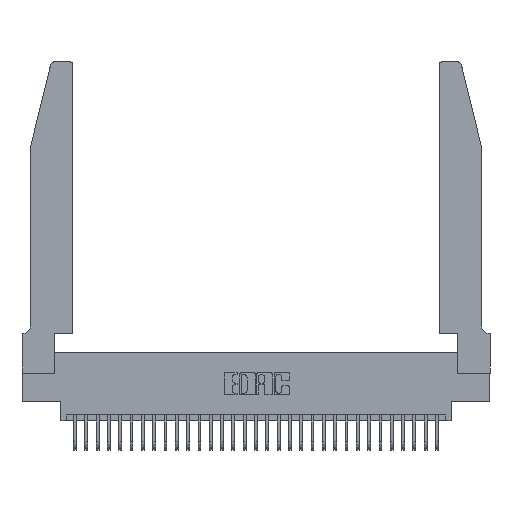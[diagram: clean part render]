
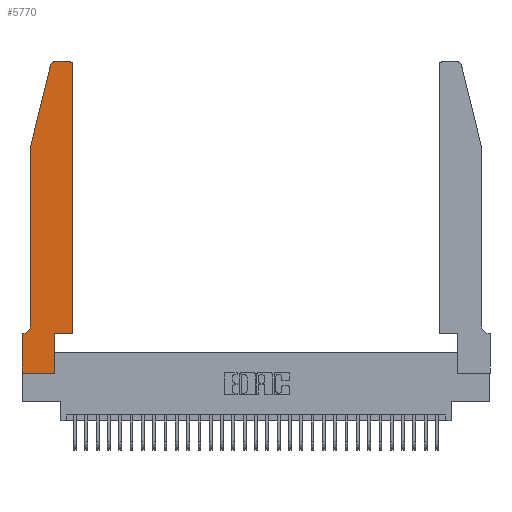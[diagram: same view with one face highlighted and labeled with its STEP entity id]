
A CAD part, top view. The second image highlights one B-rep face of the part: STEP entity #5770.
In plain terms, the highlighted planar face has unit normal (0, 0, 1).
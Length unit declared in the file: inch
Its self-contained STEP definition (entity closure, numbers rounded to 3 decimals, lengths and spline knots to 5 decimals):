
#1245 = DIRECTION ( 'NONE',  ( 0., 0., 1. ) ) ;
#2694 = EDGE_CURVE ( 'NONE', #26401, #29841, #24893, .T. ) ;
#2951 = CARTESIAN_POINT ( 'NONE',  ( 0., 0.35, 0.37 ) ) ;
#3336 = VECTOR ( 'NONE', #12911, 39.37008 ) ;
#3578 = VECTOR ( 'NONE', #28390, 39.37008 ) ;
#3881 = CARTESIAN_POINT ( 'NONE',  ( 0.284, 2.72, 0.37 ) ) ;
#3913 = ORIENTED_EDGE ( 'NONE', *, *, #16395, .T. ) ;
#3975 = CARTESIAN_POINT ( 'NONE',  ( 0.0755, 2., 0.37 ) ) ;
#4377 = VERTEX_POINT ( 'NONE', #7803 ) ;
#4879 = VERTEX_POINT ( 'NONE', #11976 ) ;
#4932 = EDGE_CURVE ( 'NONE', #25127, #19645, #4998, .T. ) ;
#4998 = LINE ( 'NONE', #29160, #28891 ) ;
#5212 = LINE ( 'NONE', #28103, #22792 ) ;
#5770 = ADVANCED_FACE ( 'NONE', ( #29551 ), #13381, .T. ) ;
#6280 = VECTOR ( 'NONE', #24021, 39.37008 ) ;
#6378 = DIRECTION ( 'NONE',  ( 1., 0., 0. ) ) ;
#6583 = VECTOR ( 'NONE', #12185, 39.37008 ) ;
#7130 = CARTESIAN_POINT ( 'NONE',  ( 0.4505, 0.35, 0.37 ) ) ;
#7392 = EDGE_CURVE ( 'NONE', #23771, #16984, #7540, .T. ) ;
#7540 = LINE ( 'NONE', #20444, #13159 ) ;
#7803 = CARTESIAN_POINT ( 'NONE',  ( 0.25487, 2.72718, 0.37 ) ) ;
#7874 = DIRECTION ( 'NONE',  ( 1., 0., 0. ) ) ;
#8365 = ORIENTED_EDGE ( 'NONE', *, *, #27937, .T. ) ;
#8763 = VERTEX_POINT ( 'NONE', #24655 ) ;
#8790 = ORIENTED_EDGE ( 'NONE', *, *, #21338, .T. ) ;
#9277 = EDGE_CURVE ( 'NONE', #28345, #19452, #19007, .T. ) ;
#9812 = ORIENTED_EDGE ( 'NONE', *, *, #30219, .T. ) ;
#10807 = CARTESIAN_POINT ( 'NONE',  ( 0.4505, 2.72, 0.37 ) ) ;
#11899 = CARTESIAN_POINT ( 'NONE',  ( 0.0055, 0.42, 0.37 ) ) ;
#11976 = CARTESIAN_POINT ( 'NONE',  ( 0.2865, 0., 0.37 ) ) ;
#12040 = AXIS2_PLACEMENT_3D ( 'NONE', #11899, #28498, #14314 ) ;
#12082 = CARTESIAN_POINT ( 'NONE',  ( 0.0755, 2., 0.37 ) ) ;
#12167 = ORIENTED_EDGE ( 'NONE', *, *, #15020, .T. ) ;
#12185 = DIRECTION ( 'NONE',  ( -0.239, -0.971, 0. ) ) ;
#12822 = DIRECTION ( 'NONE',  ( 0., 0., 1. ) ) ;
#12884 = CARTESIAN_POINT ( 'NONE',  ( 0.4205, 2.75, 0.37 ) ) ;
#12911 = DIRECTION ( 'NONE',  ( 0., 1., 0. ) ) ;
#13159 = VECTOR ( 'NONE', #15753, 39.37008 ) ;
#13200 = ORIENTED_EDGE ( 'NONE', *, *, #26315, .T. ) ;
#13381 = PLANE ( 'NONE',  #23855 ) ;
#13906 = DIRECTION ( 'NONE',  ( 1., 0., 0. ) ) ;
#14314 = DIRECTION ( 'NONE',  ( -1., 0., 0. ) ) ;
#15020 = EDGE_CURVE ( 'NONE', #16984, #4879, #5212, .T. ) ;
#15743 = CARTESIAN_POINT ( 'NONE',  ( 0., 0.35, 0.37 ) ) ;
#15753 = DIRECTION ( 'NONE',  ( 0., -1., 0. ) ) ;
#16395 = EDGE_CURVE ( 'NONE', #4879, #25127, #21953, .T. ) ;
#16886 = CARTESIAN_POINT ( 'NONE',  ( 0.0755, 2., 0.37 ) ) ;
#16984 = VERTEX_POINT ( 'NONE', #19026 ) ;
#17107 = DIRECTION ( 'NONE',  ( -1., 0., 0. ) ) ;
#17179 = ORIENTED_EDGE ( 'NONE', *, *, #30887, .T. ) ;
#17757 = AXIS2_PLACEMENT_3D ( 'NONE', #3881, #20674, #6378 ) ;
#17767 = DIRECTION ( 'NONE',  ( -1., 0., 0. ) ) ;
#18003 = ORIENTED_EDGE ( 'NONE', *, *, #4932, .T. ) ;
#18057 = LINE ( 'NONE', #28904, #29170 ) ;
#18135 = DIRECTION ( 'NONE',  ( 1., 0., 0. ) ) ;
#18404 = AXIS2_PLACEMENT_3D ( 'NONE', #27058, #12822, #29395 ) ;
#18415 = VECTOR ( 'NONE', #17767, 39.37008 ) ;
#18959 = CARTESIAN_POINT ( 'NONE',  ( 0.2865, 0.35, 0.37 ) ) ;
#19007 = LINE ( 'NONE', #16886, #6280 ) ;
#19026 = CARTESIAN_POINT ( 'NONE',  ( 0., 0., 0.37 ) ) ;
#19164 = LINE ( 'NONE', #24917, #18415 ) ;
#19452 = VERTEX_POINT ( 'NONE', #30192 ) ;
#19645 = VERTEX_POINT ( 'NONE', #7130 ) ;
#19869 = VERTEX_POINT ( 'NONE', #22086 ) ;
#19970 = CARTESIAN_POINT ( 'NONE',  ( 0.4505, 0.35, 0.37 ) ) ;
#20444 = CARTESIAN_POINT ( 'NONE',  ( 0., 0., 0.37 ) ) ;
#20674 = DIRECTION ( 'NONE',  ( 0., 0., 1. ) ) ;
#20768 = LINE ( 'NONE', #12082, #6583 ) ;
#21139 = ORIENTED_EDGE ( 'NONE', *, *, #7392, .T. ) ;
#21338 = EDGE_CURVE ( 'NONE', #19869, #4377, #25795, .T. ) ;
#21722 = LINE ( 'NONE', #19970, #3336 ) ;
#21953 = LINE ( 'NONE', #18959, #3578 ) ;
#22086 = CARTESIAN_POINT ( 'NONE',  ( 0.284, 2.75, 0.37 ) ) ;
#22792 = VECTOR ( 'NONE', #13906, 39.37008 ) ;
#22816 = CARTESIAN_POINT ( 'NONE',  ( 0.2865, 0.35, 0.37 ) ) ;
#23314 = EDGE_LOOP ( 'NONE', ( #13200, #8790, #8365, #26783, #30482, #9812, #21139, #12167, #3913, #18003, #17179, #24333 ) ) ;
#23573 = EDGE_CURVE ( 'NONE', #19452, #8763, #30414, .T. ) ;
#23771 = VERTEX_POINT ( 'NONE', #2951 ) ;
#23855 = AXIS2_PLACEMENT_3D ( 'NONE', #15743, #1245, #18135 ) ;
#24021 = DIRECTION ( 'NONE',  ( 0., -1., 0. ) ) ;
#24333 = ORIENTED_EDGE ( 'NONE', *, *, #2694, .T. ) ;
#24655 = CARTESIAN_POINT ( 'NONE',  ( 0.0055, 0.35, 0.37 ) ) ;
#24893 = CIRCLE ( 'NONE', #18404, 0.03 ) ;
#24917 = CARTESIAN_POINT ( 'NONE',  ( 0.2605, 2.75, 0.37 ) ) ;
#25127 = VERTEX_POINT ( 'NONE', #22816 ) ;
#25795 = CIRCLE ( 'NONE', #17757, 0.03 ) ;
#26315 = EDGE_CURVE ( 'NONE', #29841, #19869, #19164, .T. ) ;
#26401 = VERTEX_POINT ( 'NONE', #10807 ) ;
#26783 = ORIENTED_EDGE ( 'NONE', *, *, #9277, .T. ) ;
#27058 = CARTESIAN_POINT ( 'NONE',  ( 0.4205, 2.72, 0.37 ) ) ;
#27937 = EDGE_CURVE ( 'NONE', #4377, #28345, #20768, .T. ) ;
#28103 = CARTESIAN_POINT ( 'NONE',  ( 0., 0., 0.37 ) ) ;
#28345 = VERTEX_POINT ( 'NONE', #3975 ) ;
#28390 = DIRECTION ( 'NONE',  ( 0., 1., 0. ) ) ;
#28498 = DIRECTION ( 'NONE',  ( 0., 0., -1. ) ) ;
#28891 = VECTOR ( 'NONE', #7874, 39.37008 ) ;
#28904 = CARTESIAN_POINT ( 'NONE',  ( 0.0755, 0.35, 0.37 ) ) ;
#29160 = CARTESIAN_POINT ( 'NONE',  ( 0.4505, 0.35, 0.37 ) ) ;
#29170 = VECTOR ( 'NONE', #17107, 39.37008 ) ;
#29395 = DIRECTION ( 'NONE',  ( 1., 0., 0. ) ) ;
#29551 = FACE_OUTER_BOUND ( 'NONE', #23314, .T. ) ;
#29841 = VERTEX_POINT ( 'NONE', #12884 ) ;
#30192 = CARTESIAN_POINT ( 'NONE',  ( 0.0755, 0.42, 0.37 ) ) ;
#30219 = EDGE_CURVE ( 'NONE', #8763, #23771, #18057, .T. ) ;
#30414 = CIRCLE ( 'NONE', #12040, 0.07 ) ;
#30482 = ORIENTED_EDGE ( 'NONE', *, *, #23573, .T. ) ;
#30887 = EDGE_CURVE ( 'NONE', #19645, #26401, #21722, .T. ) ;
